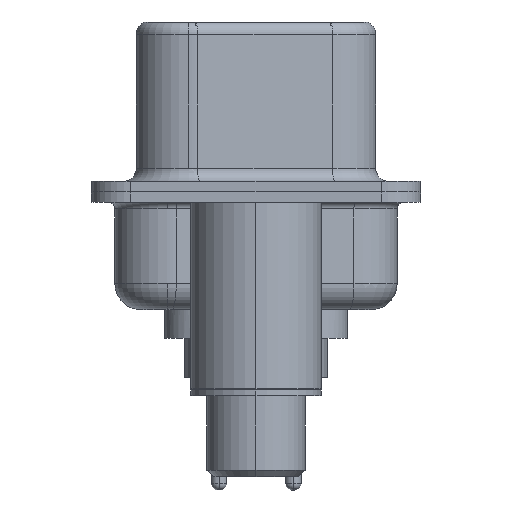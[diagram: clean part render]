
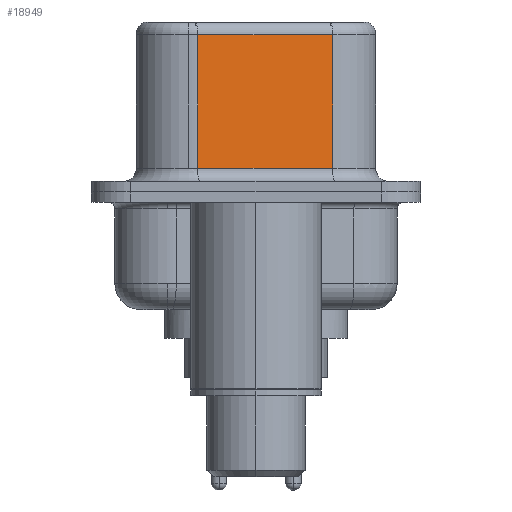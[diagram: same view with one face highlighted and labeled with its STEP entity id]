
A CAD part, left-side view. The second image highlights one B-rep face of the part: STEP entity #18949.
In plain terms, the highlighted planar face has unit normal (-0.985, -0.174, 0).
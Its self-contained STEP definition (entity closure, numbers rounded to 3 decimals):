
#35 = DIRECTION ( 'NONE',  ( -0.174, 0.985, 0. ) ) ;
#135 = VERTEX_POINT ( 'NONE', #5244 ) ;
#780 = EDGE_CURVE ( 'NONE', #1970, #7063, #19146, .T. ) ;
#1320 = CARTESIAN_POINT ( 'NONE',  ( 4.58, -2.927, 6.52 ) ) ;
#1953 = ORIENTED_EDGE ( 'NONE', *, *, #780, .T. ) ;
#1970 = VERTEX_POINT ( 'NONE', #14782 ) ;
#2955 = ORIENTED_EDGE ( 'NONE', *, *, #9454, .T. ) ;
#3253 = DIRECTION ( 'NONE',  ( 0., 0., -1. ) ) ;
#3705 = EDGE_LOOP ( 'NONE', ( #8142, #1953, #13395, #2955 ) ) ;
#4143 = CARTESIAN_POINT ( 'NONE',  ( 4.58, -2.927, 0.9 ) ) ;
#4579 = EDGE_CURVE ( 'NONE', #7063, #14419, #16079, .T. ) ;
#5106 = DIRECTION ( 'NONE',  ( -0.174, 0.985, 0. ) ) ;
#5244 = CARTESIAN_POINT ( 'NONE',  ( 4.58, -2.927, 0.9 ) ) ;
#6294 = CARTESIAN_POINT ( 'NONE',  ( 4.58, -2.927, 6.02 ) ) ;
#6863 = VECTOR ( 'NONE', #5106, 1000. ) ;
#7063 = VERTEX_POINT ( 'NONE', #14374 ) ;
#7199 = VECTOR ( 'NONE', #15084, 1000. ) ;
#7588 = CARTESIAN_POINT ( 'NONE',  ( 4.58, -2.927, 6.52 ) ) ;
#8142 = ORIENTED_EDGE ( 'NONE', *, *, #10496, .F. ) ;
#8377 = VECTOR ( 'NONE', #3253, 1000. ) ;
#8724 = DIRECTION ( 'NONE',  ( 0.174, -0.985, 0. ) ) ;
#9114 = DIRECTION ( 'NONE',  ( 0.985, 0.174, 0. ) ) ;
#9304 = CARTESIAN_POINT ( 'NONE',  ( 3.67, 2.233, 6.52 ) ) ;
#9454 = EDGE_CURVE ( 'NONE', #14419, #135, #18554, .T. ) ;
#10136 = CARTESIAN_POINT ( 'NONE',  ( 3.67, 2.233, 0.9 ) ) ;
#10496 = EDGE_CURVE ( 'NONE', #1970, #135, #11272, .T. ) ;
#11272 = LINE ( 'NONE', #1320, #7199 ) ;
#13395 = ORIENTED_EDGE ( 'NONE', *, *, #4579, .T. ) ;
#14374 = CARTESIAN_POINT ( 'NONE',  ( 3.67, 2.233, 6.02 ) ) ;
#14419 = VERTEX_POINT ( 'NONE', #10136 ) ;
#14440 = VECTOR ( 'NONE', #8724, 1000. ) ;
#14782 = CARTESIAN_POINT ( 'NONE',  ( 4.58, -2.927, 6.02 ) ) ;
#15084 = DIRECTION ( 'NONE',  ( 0., 0., -1. ) ) ;
#16079 = LINE ( 'NONE', #9304, #8377 ) ;
#16104 = FACE_OUTER_BOUND ( 'NONE', #3705, .T. ) ;
#16820 = PLANE ( 'NONE',  #18604 ) ;
#18554 = LINE ( 'NONE', #4143, #14440 ) ;
#18604 = AXIS2_PLACEMENT_3D ( 'NONE', #7588, #9114, #35 ) ;
#18949 = ADVANCED_FACE ( 'NONE', ( #16104 ), #16820, .F. ) ;
#19146 = LINE ( 'NONE', #6294, #6863 ) ;
